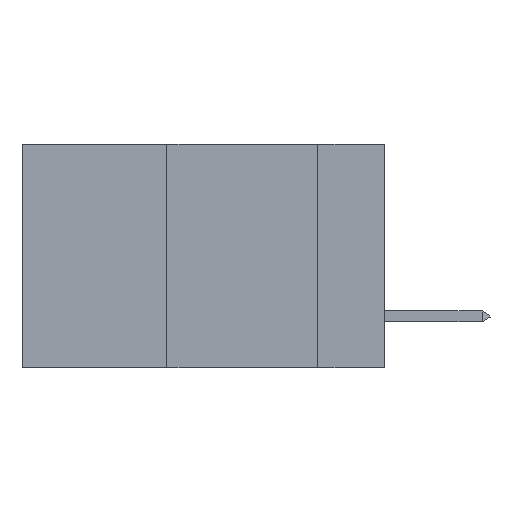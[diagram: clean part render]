
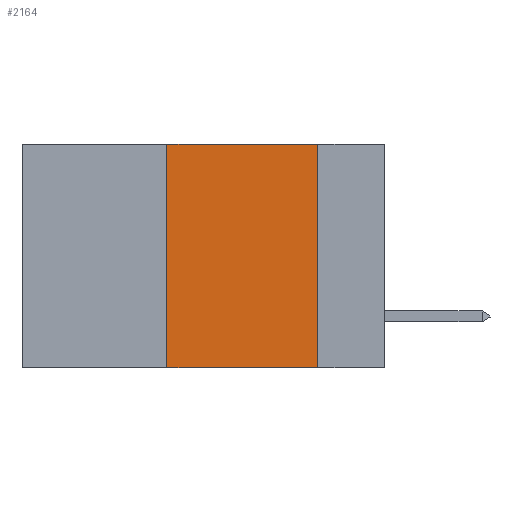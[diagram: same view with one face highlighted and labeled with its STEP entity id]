
A CAD part, left-side view. The second image highlights one B-rep face of the part: STEP entity #2164.
In plain terms, the highlighted planar face has unit normal (-1, 0, 0).
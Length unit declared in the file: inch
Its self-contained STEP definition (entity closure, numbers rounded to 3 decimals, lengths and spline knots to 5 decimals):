
#1273 = EDGE_LOOP ( 'NONE', ( #6586, #15976, #5637, #11662 ) ) ;
#1475 = AXIS2_PLACEMENT_3D ( 'NONE', #5747, #17746, #9218 ) ;
#2164 = ADVANCED_FACE ( 'NONE', ( #8051 ), #17672, .F. ) ;
#4659 = CARTESIAN_POINT ( 'NONE',  ( 0., 0.6, -0.37 ) ) ;
#4867 = CARTESIAN_POINT ( 'NONE',  ( 0., 0.11, 0. ) ) ;
#4988 = EDGE_CURVE ( 'NONE', #14713, #21871, #11841, .T. ) ;
#5637 = ORIENTED_EDGE ( 'NONE', *, *, #4988, .F. ) ;
#5747 = CARTESIAN_POINT ( 'NONE',  ( 0., 0.6, 0. ) ) ;
#6586 = ORIENTED_EDGE ( 'NONE', *, *, #22364, .F. ) ;
#6640 = DIRECTION ( 'NONE',  ( 0., 0., -1. ) ) ;
#7764 = CARTESIAN_POINT ( 'NONE',  ( 0., 0.36, 0. ) ) ;
#8051 = FACE_OUTER_BOUND ( 'NONE', #1273, .T. ) ;
#9218 = DIRECTION ( 'NONE',  ( 0., 0., -1. ) ) ;
#9987 = DIRECTION ( 'NONE',  ( 0., -1., 0. ) ) ;
#10197 = VECTOR ( 'NONE', #11191, 39.37008 ) ;
#10199 = EDGE_CURVE ( 'NONE', #21871, #22321, #17853, .T. ) ;
#10773 = DIRECTION ( 'NONE',  ( 0., -1., 0. ) ) ;
#11191 = DIRECTION ( 'NONE',  ( 0., 0., 1. ) ) ;
#11662 = ORIENTED_EDGE ( 'NONE', *, *, #21615, .T. ) ;
#11841 = LINE ( 'NONE', #7764, #10197 ) ;
#13237 = VECTOR ( 'NONE', #10773, 39.37008 ) ;
#14713 = VERTEX_POINT ( 'NONE', #19645 ) ;
#14972 = VERTEX_POINT ( 'NONE', #20490 ) ;
#15976 = ORIENTED_EDGE ( 'NONE', *, *, #10199, .F. ) ;
#16296 = LINE ( 'NONE', #4659, #21490 ) ;
#17177 = CARTESIAN_POINT ( 'NONE',  ( 0., 0.11, 0. ) ) ;
#17672 = PLANE ( 'NONE',  #1475 ) ;
#17746 = DIRECTION ( 'NONE',  ( 1., 0., 0. ) ) ;
#17853 = LINE ( 'NONE', #18021, #13237 ) ;
#17899 = LINE ( 'NONE', #4867, #18191 ) ;
#18021 = CARTESIAN_POINT ( 'NONE',  ( 0., 0.6, 0. ) ) ;
#18191 = VECTOR ( 'NONE', #6640, 39.37008 ) ;
#19645 = CARTESIAN_POINT ( 'NONE',  ( 0., 0.36, -0.37 ) ) ;
#20490 = CARTESIAN_POINT ( 'NONE',  ( 0., 0.11, -0.37 ) ) ;
#21079 = CARTESIAN_POINT ( 'NONE',  ( 0., 0.36, 0. ) ) ;
#21490 = VECTOR ( 'NONE', #9987, 39.37008 ) ;
#21615 = EDGE_CURVE ( 'NONE', #14713, #14972, #16296, .T. ) ;
#21871 = VERTEX_POINT ( 'NONE', #21079 ) ;
#22321 = VERTEX_POINT ( 'NONE', #17177 ) ;
#22364 = EDGE_CURVE ( 'NONE', #22321, #14972, #17899, .T. ) ;
